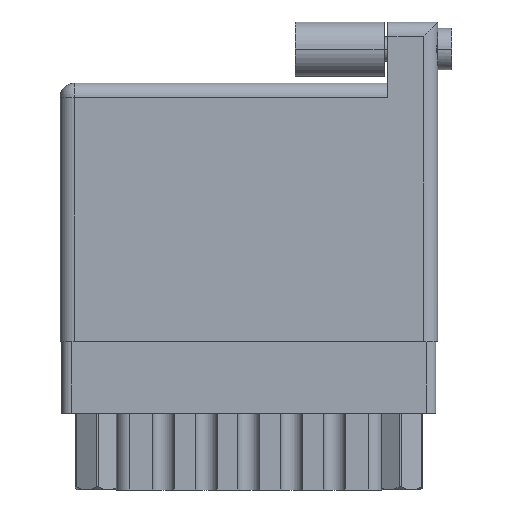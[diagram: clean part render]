
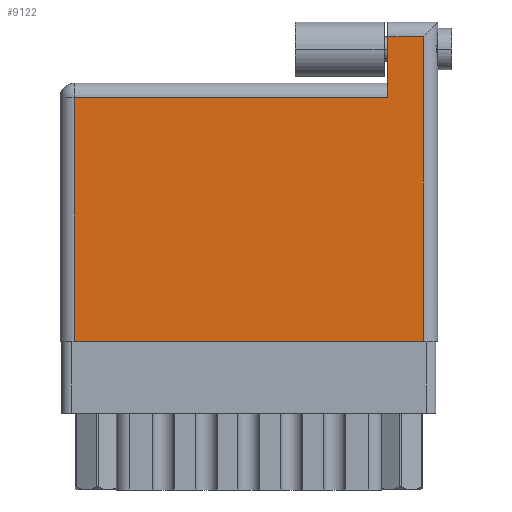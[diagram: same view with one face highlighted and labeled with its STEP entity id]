
A CAD part, front view. The second image highlights one B-rep face of the part: STEP entity #9122.
In plain terms, the highlighted face is planar.
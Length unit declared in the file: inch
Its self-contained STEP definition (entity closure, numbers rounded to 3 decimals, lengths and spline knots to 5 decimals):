
#476 = LINE ( 'NONE', #32379, #24708 ) ;
#733 = VECTOR ( 'NONE', #26810, 39.37008 ) ;
#1841 = VECTOR ( 'NONE', #14561, 39.37008 ) ;
#2091 = ORIENTED_EDGE ( 'NONE', *, *, #11329, .T. ) ;
#2522 = CARTESIAN_POINT ( 'NONE',  ( 0., 1.07, 0. ) ) ;
#2825 = CARTESIAN_POINT ( 'NONE',  ( 0.05, 0., 0. ) ) ;
#2940 = VERTEX_POINT ( 'NONE', #17072 ) ;
#3095 = CARTESIAN_POINT ( 'NONE',  ( 0., 0.856, 0. ) ) ;
#3698 = VERTEX_POINT ( 'NONE', #27218 ) ;
#5372 = EDGE_LOOP ( 'NONE', ( #22407, #28564, #20452, #2091, #9367, #30736 ) ) ;
#6616 = CARTESIAN_POINT ( 'NONE',  ( 0., 0., 0. ) ) ;
#8043 = CARTESIAN_POINT ( 'NONE',  ( 1.275, 0., 0. ) ) ;
#9122 = ADVANCED_FACE ( 'NONE', ( #27992 ), #27643, .F. ) ;
#9367 = ORIENTED_EDGE ( 'NONE', *, *, #15845, .T. ) ;
#11329 = EDGE_CURVE ( 'NONE', #3698, #28784, #476, .T. ) ;
#11400 = LINE ( 'NONE', #3095, #16836 ) ;
#11621 = DIRECTION ( 'NONE',  ( -1., 0., 0. ) ) ;
#12140 = AXIS2_PLACEMENT_3D ( 'NONE', #28333, #16901, #11621 ) ;
#13001 = VERTEX_POINT ( 'NONE', #8043 ) ;
#14561 = DIRECTION ( 'NONE',  ( 1., 0., 0. ) ) ;
#15845 = EDGE_CURVE ( 'NONE', #28784, #2940, #11400, .T. ) ;
#16275 = DIRECTION ( 'NONE',  ( 0., 1., 0. ) ) ;
#16836 = VECTOR ( 'NONE', #32892, 39.37008 ) ;
#16901 = DIRECTION ( 'NONE',  ( 0., 0., -1. ) ) ;
#17072 = CARTESIAN_POINT ( 'NONE',  ( 0.05, 0.856, 0. ) ) ;
#17194 = LINE ( 'NONE', #6616, #1841 ) ;
#18334 = VECTOR ( 'NONE', #34618, 39.37008 ) ;
#18907 = CARTESIAN_POINT ( 'NONE',  ( 1.275, 1.07, 0. ) ) ;
#18908 = LINE ( 'NONE', #29672, #31211 ) ;
#20452 = ORIENTED_EDGE ( 'NONE', *, *, #33015, .T. ) ;
#20551 = EDGE_CURVE ( 'NONE', #22939, #13001, #17194, .T. ) ;
#20936 = EDGE_CURVE ( 'NONE', #2940, #22939, #29642, .T. ) ;
#22204 = CARTESIAN_POINT ( 'NONE',  ( 1.15, 0.856, 0. ) ) ;
#22407 = ORIENTED_EDGE ( 'NONE', *, *, #20551, .T. ) ;
#22939 = VERTEX_POINT ( 'NONE', #23483 ) ;
#23112 = VERTEX_POINT ( 'NONE', #18907 ) ;
#23483 = CARTESIAN_POINT ( 'NONE',  ( 0.05, 0., 0. ) ) ;
#24708 = VECTOR ( 'NONE', #27093, 39.37008 ) ;
#26810 = DIRECTION ( 'NONE',  ( 0., -1., 0. ) ) ;
#27093 = DIRECTION ( 'NONE',  ( 0., -1., 0. ) ) ;
#27218 = CARTESIAN_POINT ( 'NONE',  ( 1.15, 1.07, 0. ) ) ;
#27643 = PLANE ( 'NONE',  #12140 ) ;
#27992 = FACE_OUTER_BOUND ( 'NONE', #5372, .T. ) ;
#28333 = CARTESIAN_POINT ( 'NONE',  ( 0., 0.906, 0. ) ) ;
#28564 = ORIENTED_EDGE ( 'NONE', *, *, #32155, .T. ) ;
#28784 = VERTEX_POINT ( 'NONE', #22204 ) ;
#29642 = LINE ( 'NONE', #2825, #733 ) ;
#29672 = CARTESIAN_POINT ( 'NONE',  ( 1.275, 1.12, 0. ) ) ;
#30736 = ORIENTED_EDGE ( 'NONE', *, *, #20936, .T. ) ;
#31211 = VECTOR ( 'NONE', #16275, 39.37008 ) ;
#32155 = EDGE_CURVE ( 'NONE', #13001, #23112, #18908, .T. ) ;
#32306 = LINE ( 'NONE', #2522, #18334 ) ;
#32379 = CARTESIAN_POINT ( 'NONE',  ( 1.15, 1.12, 0. ) ) ;
#32892 = DIRECTION ( 'NONE',  ( -1., 0., 0. ) ) ;
#33015 = EDGE_CURVE ( 'NONE', #23112, #3698, #32306, .T. ) ;
#34618 = DIRECTION ( 'NONE',  ( -1., 0., 0. ) ) ;
